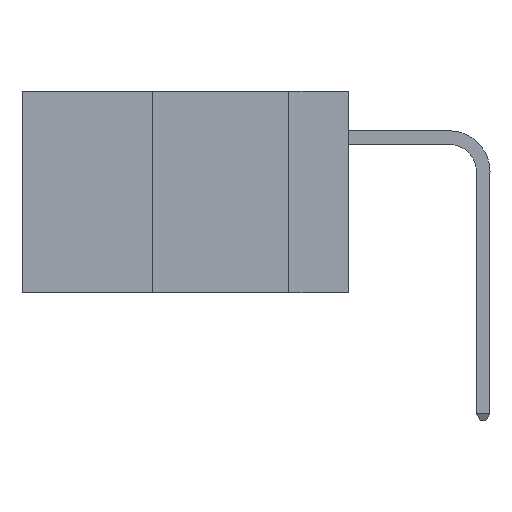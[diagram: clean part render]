
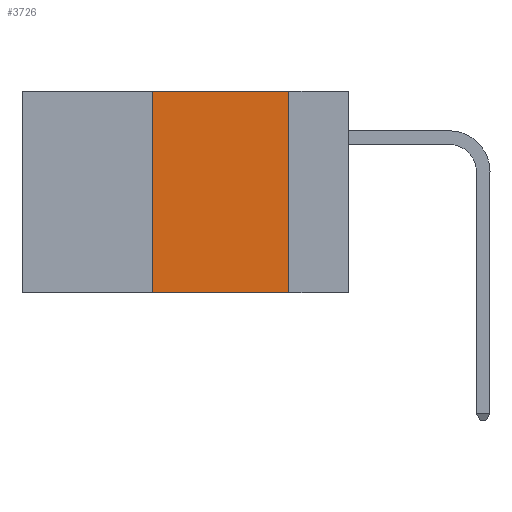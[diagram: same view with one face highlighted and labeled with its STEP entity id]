
A CAD part, left-side view. The second image highlights one B-rep face of the part: STEP entity #3726.
In plain terms, the highlighted planar face has unit normal (-1, 0, 0).
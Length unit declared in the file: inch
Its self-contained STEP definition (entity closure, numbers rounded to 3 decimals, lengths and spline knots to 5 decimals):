
#1786 = LINE ( 'NONE', #17128, #18258 ) ;
#3211 = EDGE_CURVE ( 'NONE', #28741, #23595, #1786, .T. ) ;
#3726 = ADVANCED_FACE ( 'NONE', ( #22385 ), #18106, .F. ) ;
#4355 = EDGE_CURVE ( 'NONE', #23595, #22793, #16684, .T. ) ;
#5883 = VECTOR ( 'NONE', #15027, 39.37008 ) ;
#6869 = DIRECTION ( 'NONE',  ( 1., 0., 0. ) ) ;
#10040 = CARTESIAN_POINT ( 'NONE',  ( 0., 0.11, 0. ) ) ;
#10190 = CARTESIAN_POINT ( 'NONE',  ( 0., 0.11, 0. ) ) ;
#11414 = CARTESIAN_POINT ( 'NONE',  ( 0., 0.36, 0. ) ) ;
#11435 = VECTOR ( 'NONE', #19867, 39.37008 ) ;
#11464 = DIRECTION ( 'NONE',  ( 0., 0., -1. ) ) ;
#12722 = ORIENTED_EDGE ( 'NONE', *, *, #14870, .T. ) ;
#12964 = CARTESIAN_POINT ( 'NONE',  ( 0., 0.36, -0.37 ) ) ;
#14870 = EDGE_CURVE ( 'NONE', #26337, #22793, #24588, .T. ) ;
#15027 = DIRECTION ( 'NONE',  ( 0., 0., 1. ) ) ;
#15730 = ORIENTED_EDGE ( 'NONE', *, *, #4355, .F. ) ;
#15879 = CARTESIAN_POINT ( 'NONE',  ( 0., 0.6, -0.37 ) ) ;
#15896 = CARTESIAN_POINT ( 'NONE',  ( 0., 0.6, 0. ) ) ;
#16684 = LINE ( 'NONE', #10040, #20235 ) ;
#17128 = CARTESIAN_POINT ( 'NONE',  ( 0., 0.6, 0. ) ) ;
#17517 = CARTESIAN_POINT ( 'NONE',  ( 0., 0.36, 0. ) ) ;
#18106 = PLANE ( 'NONE',  #19289 ) ;
#18258 = VECTOR ( 'NONE', #19493, 39.37008 ) ;
#18858 = ORIENTED_EDGE ( 'NONE', *, *, #18874, .F. ) ;
#18874 = EDGE_CURVE ( 'NONE', #26337, #28741, #26392, .T. ) ;
#19048 = DIRECTION ( 'NONE',  ( 0., 0., -1. ) ) ;
#19289 = AXIS2_PLACEMENT_3D ( 'NONE', #15896, #6869, #11464 ) ;
#19493 = DIRECTION ( 'NONE',  ( 0., -1., 0. ) ) ;
#19572 = ORIENTED_EDGE ( 'NONE', *, *, #3211, .F. ) ;
#19867 = DIRECTION ( 'NONE',  ( 0., -1., 0. ) ) ;
#20235 = VECTOR ( 'NONE', #19048, 39.37008 ) ;
#22385 = FACE_OUTER_BOUND ( 'NONE', #23749, .T. ) ;
#22793 = VERTEX_POINT ( 'NONE', #23249 ) ;
#23249 = CARTESIAN_POINT ( 'NONE',  ( 0., 0.11, -0.37 ) ) ;
#23595 = VERTEX_POINT ( 'NONE', #10190 ) ;
#23749 = EDGE_LOOP ( 'NONE', ( #15730, #19572, #18858, #12722 ) ) ;
#24588 = LINE ( 'NONE', #15879, #11435 ) ;
#26337 = VERTEX_POINT ( 'NONE', #12964 ) ;
#26392 = LINE ( 'NONE', #17517, #5883 ) ;
#28741 = VERTEX_POINT ( 'NONE', #11414 ) ;
